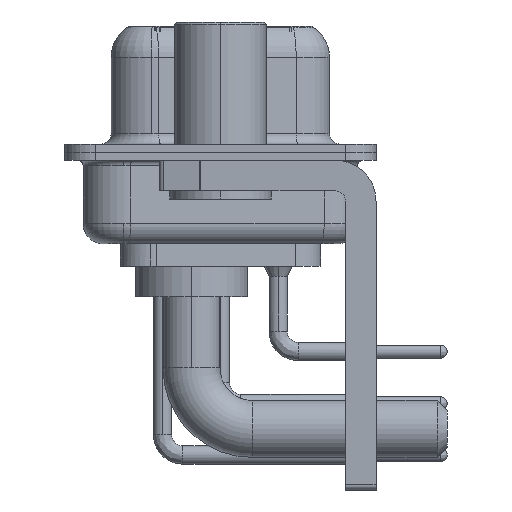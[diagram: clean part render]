
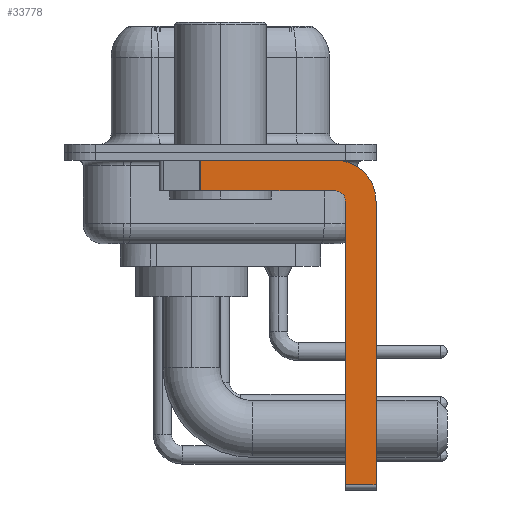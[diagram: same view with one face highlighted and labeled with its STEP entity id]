
A CAD part, left-side view. The second image highlights one B-rep face of the part: STEP entity #33778.
In plain terms, the highlighted planar face has unit normal (-1, 0, 0).
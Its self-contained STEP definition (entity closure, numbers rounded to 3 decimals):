
#527 = DIRECTION ( 'NONE',  ( 1., 0., 0. ) ) ;
#634 = CARTESIAN_POINT ( 'NONE',  ( -2.9, -7.65, -16.35 ) ) ;
#1043 = DIRECTION ( 'NONE',  ( 0., 0., 1. ) ) ;
#1093 = VERTEX_POINT ( 'NONE', #34853 ) ;
#1287 = VECTOR ( 'NONE', #6696, 1000. ) ;
#2428 = VECTOR ( 'NONE', #1043, 1000. ) ;
#2606 = EDGE_LOOP ( 'NONE', ( #27021, #13203, #17818, #6210, #12797, #3290, #4169, #5434 ) ) ;
#2852 = DIRECTION ( 'NONE',  ( 0., 0., -1. ) ) ;
#3290 = ORIENTED_EDGE ( 'NONE', *, *, #14242, .T. ) ;
#3414 = VERTEX_POINT ( 'NONE', #3955 ) ;
#3470 = DIRECTION ( 'NONE',  ( 0., 0., -1. ) ) ;
#3825 = FACE_OUTER_BOUND ( 'NONE', #2606, .T. ) ;
#3955 = CARTESIAN_POINT ( 'NONE',  ( -2.9, -7.65, -2.4 ) ) ;
#4169 = ORIENTED_EDGE ( 'NONE', *, *, #8654, .F. ) ;
#5434 = ORIENTED_EDGE ( 'NONE', *, *, #34398, .F. ) ;
#5491 = EDGE_CURVE ( 'NONE', #11460, #1093, #10617, .T. ) ;
#6210 = ORIENTED_EDGE ( 'NONE', *, *, #32726, .F. ) ;
#6535 = CARTESIAN_POINT ( 'NONE',  ( -2.9, -5.65, -2.4 ) ) ;
#6696 = DIRECTION ( 'NONE',  ( 0., 0., -1. ) ) ;
#7465 = DIRECTION ( 'NONE',  ( 0., 1., 0. ) ) ;
#7919 = CARTESIAN_POINT ( 'NONE',  ( -2.9, -5.65, -1.9 ) ) ;
#8654 = EDGE_CURVE ( 'NONE', #3414, #25587, #21226, .T. ) ;
#9676 = CIRCLE ( 'NONE', #19768, 2. ) ;
#10617 = LINE ( 'NONE', #33151, #18939 ) ;
#10831 = AXIS2_PLACEMENT_3D ( 'NONE', #11586, #527, #3470 ) ;
#11340 = VERTEX_POINT ( 'NONE', #30083 ) ;
#11460 = VERTEX_POINT ( 'NONE', #7919 ) ;
#11586 = CARTESIAN_POINT ( 'NONE',  ( -2.9, -5.65, -2.4 ) ) ;
#12056 = DIRECTION ( 'NONE',  ( -1., 0., 0. ) ) ;
#12136 = DIRECTION ( 'NONE',  ( 0., 0., -1. ) ) ;
#12797 = ORIENTED_EDGE ( 'NONE', *, *, #16438, .F. ) ;
#13203 = ORIENTED_EDGE ( 'NONE', *, *, #30474, .T. ) ;
#13688 = EDGE_CURVE ( 'NONE', #28447, #35913, #21684, .T. ) ;
#14242 = EDGE_CURVE ( 'NONE', #11340, #25587, #27713, .T. ) ;
#16096 = CARTESIAN_POINT ( 'NONE',  ( -2.9, -5.65, -16.35 ) ) ;
#16438 = EDGE_CURVE ( 'NONE', #11340, #32154, #24096, .T. ) ;
#17818 = ORIENTED_EDGE ( 'NONE', *, *, #5491, .F. ) ;
#18939 = VECTOR ( 'NONE', #7465, 1000. ) ;
#19289 = DIRECTION ( 'NONE',  ( 1., 0., 0. ) ) ;
#19648 = DIRECTION ( 'NONE',  ( 0., -1., 0. ) ) ;
#19768 = AXIS2_PLACEMENT_3D ( 'NONE', #36074, #19289, #2852 ) ;
#21226 = LINE ( 'NONE', #32285, #30272 ) ;
#21684 = LINE ( 'NONE', #24993, #29312 ) ;
#23336 = DIRECTION ( 'NONE',  ( 0., 0., 1. ) ) ;
#23366 = CARTESIAN_POINT ( 'NONE',  ( -2.9, -6.15, -16.6 ) ) ;
#24096 = LINE ( 'NONE', #23366, #2428 ) ;
#24993 = CARTESIAN_POINT ( 'NONE',  ( -2.9, 3., -0.4 ) ) ;
#25436 = CARTESIAN_POINT ( 'NONE',  ( -2.9, -6.15, -2.4 ) ) ;
#25587 = VERTEX_POINT ( 'NONE', #634 ) ;
#25831 = CARTESIAN_POINT ( 'NONE',  ( -2.9, -5.65, -0.4 ) ) ;
#27021 = ORIENTED_EDGE ( 'NONE', *, *, #13688, .F. ) ;
#27343 = DIRECTION ( 'NONE',  ( 0., -1., 0. ) ) ;
#27713 = LINE ( 'NONE', #16096, #34697 ) ;
#28438 = CIRCLE ( 'NONE', #29035, 0.5 ) ;
#28447 = VERTEX_POINT ( 'NONE', #35959 ) ;
#28866 = LINE ( 'NONE', #31638, #1287 ) ;
#29035 = AXIS2_PLACEMENT_3D ( 'NONE', #6535, #12056, #23336 ) ;
#29312 = VECTOR ( 'NONE', #19648, 1000. ) ;
#30083 = CARTESIAN_POINT ( 'NONE',  ( -2.9, -6.15, -16.35 ) ) ;
#30272 = VECTOR ( 'NONE', #12136, 1000. ) ;
#30474 = EDGE_CURVE ( 'NONE', #28447, #1093, #28866, .T. ) ;
#31638 = CARTESIAN_POINT ( 'NONE',  ( -2.9, 0.978, -1.9 ) ) ;
#31701 = PLANE ( 'NONE',  #10831 ) ;
#32154 = VERTEX_POINT ( 'NONE', #25436 ) ;
#32285 = CARTESIAN_POINT ( 'NONE',  ( -2.9, -7.65, -2.4 ) ) ;
#32726 = EDGE_CURVE ( 'NONE', #32154, #11460, #28438, .T. ) ;
#33151 = CARTESIAN_POINT ( 'NONE',  ( -2.9, -5.65, -1.9 ) ) ;
#33778 = ADVANCED_FACE ( 'NONE', ( #3825 ), #31701, .F. ) ;
#34398 = EDGE_CURVE ( 'NONE', #35913, #3414, #9676, .T. ) ;
#34697 = VECTOR ( 'NONE', #27343, 1000. ) ;
#34853 = CARTESIAN_POINT ( 'NONE',  ( -2.9, 0.978, -1.9 ) ) ;
#35913 = VERTEX_POINT ( 'NONE', #25831 ) ;
#35959 = CARTESIAN_POINT ( 'NONE',  ( -2.9, 0.978, -0.4 ) ) ;
#36074 = CARTESIAN_POINT ( 'NONE',  ( -2.9, -5.65, -2.4 ) ) ;
